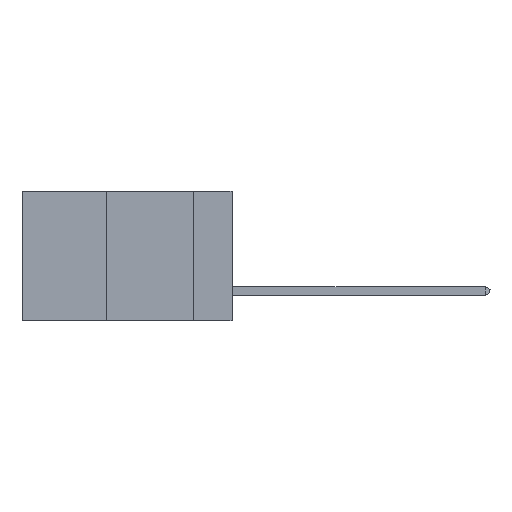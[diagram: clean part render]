
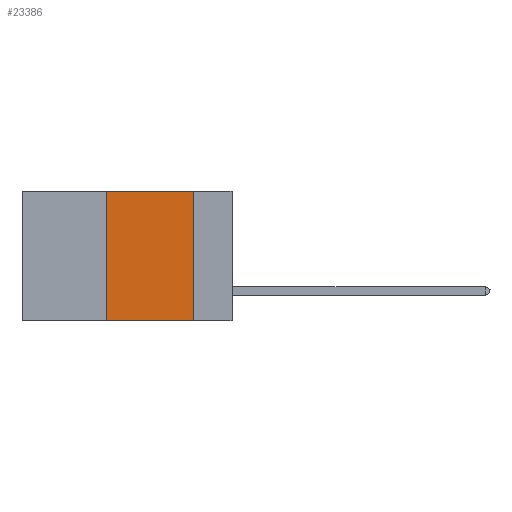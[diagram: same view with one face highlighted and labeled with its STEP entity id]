
A CAD part, left-side view. The second image highlights one B-rep face of the part: STEP entity #23386.
In plain terms, the highlighted planar face has unit normal (-1, 0, 0).
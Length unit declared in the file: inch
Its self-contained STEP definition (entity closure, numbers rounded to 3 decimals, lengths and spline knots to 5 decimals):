
#486 = EDGE_CURVE ( 'NONE', #3337, #15000, #23228, .T. ) ;
#1070 = CARTESIAN_POINT ( 'NONE',  ( 0., 0.36, 0. ) ) ;
#1090 = VECTOR ( 'NONE', #23195, 39.37008 ) ;
#2610 = LINE ( 'NONE', #22506, #3511 ) ;
#3181 = DIRECTION ( 'NONE',  ( 0., -1., 0. ) ) ;
#3337 = VERTEX_POINT ( 'NONE', #15736 ) ;
#3511 = VECTOR ( 'NONE', #13275, 39.37008 ) ;
#3853 = VERTEX_POINT ( 'NONE', #1070 ) ;
#4494 = EDGE_LOOP ( 'NONE', ( #12082, #13326, #5271, #16346 ) ) ;
#5271 = ORIENTED_EDGE ( 'NONE', *, *, #22557, .F. ) ;
#6938 = CARTESIAN_POINT ( 'NONE',  ( 0., 0.6, 0. ) ) ;
#7077 = DIRECTION ( 'NONE',  ( 0., 0., -1. ) ) ;
#7844 = CARTESIAN_POINT ( 'NONE',  ( 0., 0.11, -0.37 ) ) ;
#8292 = CARTESIAN_POINT ( 'NONE',  ( 0., 0.11, 0. ) ) ;
#9959 = CARTESIAN_POINT ( 'NONE',  ( 0., 0.6, -0.37 ) ) ;
#11353 = FACE_OUTER_BOUND ( 'NONE', #4494, .T. ) ;
#11690 = DIRECTION ( 'NONE',  ( 0., 0., -1. ) ) ;
#12082 = ORIENTED_EDGE ( 'NONE', *, *, #22904, .F. ) ;
#12348 = VECTOR ( 'NONE', #3181, 39.37008 ) ;
#13275 = DIRECTION ( 'NONE',  ( 0., 0., 1. ) ) ;
#13326 = ORIENTED_EDGE ( 'NONE', *, *, #14475, .F. ) ;
#13727 = LINE ( 'NONE', #14510, #18116 ) ;
#14369 = AXIS2_PLACEMENT_3D ( 'NONE', #17151, #22798, #11690 ) ;
#14475 = EDGE_CURVE ( 'NONE', #3853, #20912, #23972, .T. ) ;
#14510 = CARTESIAN_POINT ( 'NONE',  ( 0., 0.11, 0. ) ) ;
#15000 = VERTEX_POINT ( 'NONE', #7844 ) ;
#15736 = CARTESIAN_POINT ( 'NONE',  ( 0., 0.36, -0.37 ) ) ;
#16346 = ORIENTED_EDGE ( 'NONE', *, *, #486, .T. ) ;
#17151 = CARTESIAN_POINT ( 'NONE',  ( 0., 0.6, 0. ) ) ;
#18116 = VECTOR ( 'NONE', #7077, 39.37008 ) ;
#20912 = VERTEX_POINT ( 'NONE', #8292 ) ;
#22506 = CARTESIAN_POINT ( 'NONE',  ( 0., 0.36, 0. ) ) ;
#22557 = EDGE_CURVE ( 'NONE', #3337, #3853, #2610, .T. ) ;
#22634 = PLANE ( 'NONE',  #14369 ) ;
#22798 = DIRECTION ( 'NONE',  ( 1., 0., 0. ) ) ;
#22904 = EDGE_CURVE ( 'NONE', #20912, #15000, #13727, .T. ) ;
#23195 = DIRECTION ( 'NONE',  ( 0., -1., 0. ) ) ;
#23228 = LINE ( 'NONE', #9959, #1090 ) ;
#23386 = ADVANCED_FACE ( 'NONE', ( #11353 ), #22634, .F. ) ;
#23972 = LINE ( 'NONE', #6938, #12348 ) ;
